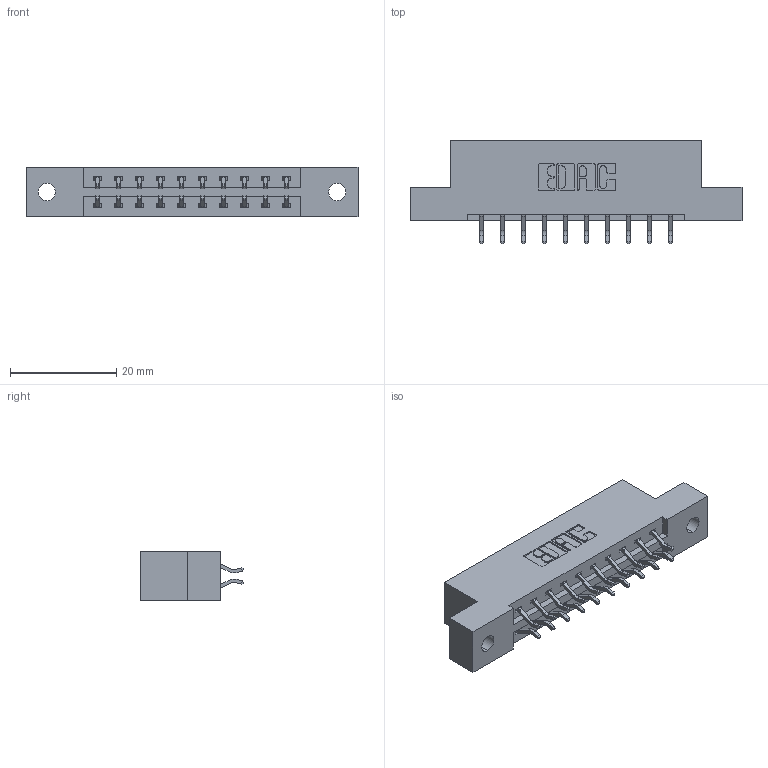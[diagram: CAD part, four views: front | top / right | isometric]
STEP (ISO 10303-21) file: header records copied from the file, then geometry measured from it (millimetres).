
FILE_DESCRIPTION (( 'STEP AP203' ), '1' );
FILE_NAME ('337-020-556-202.STEP', '2019-10-08T14:16:31', ( '' ), ( '' ), 'SwSTEP 2.0', 'SolidWorks 2016', '' );
FILE_SCHEMA (( 'CONFIG_CONTROL_DESIGN' ));
Length unit declared in the file: inch
Products named in the file (3): 345-292-001_556 Tail; 337-020-556-202; 337 Part_Flush Mounting Lugs - 0.128 Dia
Assembly tree (21 placements, depth 2):
  337-020-556-202
    337 Part_Flush Mounting Lugs - 0.128 Dia
    345-292-001_556 Tail  x20
Bounding box: 62.64 x 19.57 x 9.4 mm (x, y, z)
Volume: 6137.7 mm3; surface area: 6334 mm2
Topology: 21 solids, 21 shells, 1314 faces, 3891 edges, 2566 vertices
Faces by surface type: plane 910, cylinder 404
Entity records: 12115 total; most frequent: CARTESIAN_POINT 2082, ORIENTED_EDGE 2006, DIRECTION 1819, EDGE_CURVE 1003, VECTOR 867, LINE 867, VERTEX_POINT 666, AXIS2_PLACEMENT_3D 476
